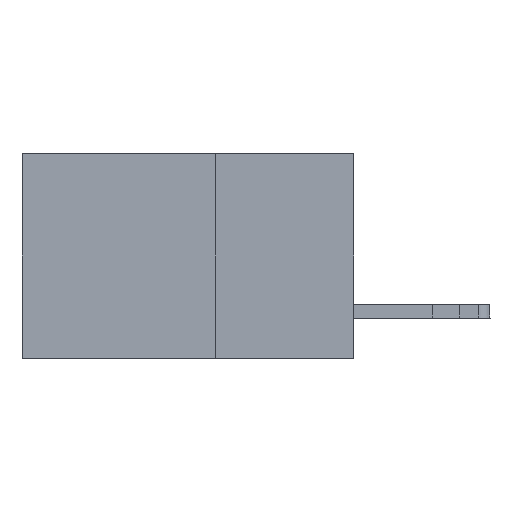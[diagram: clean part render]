
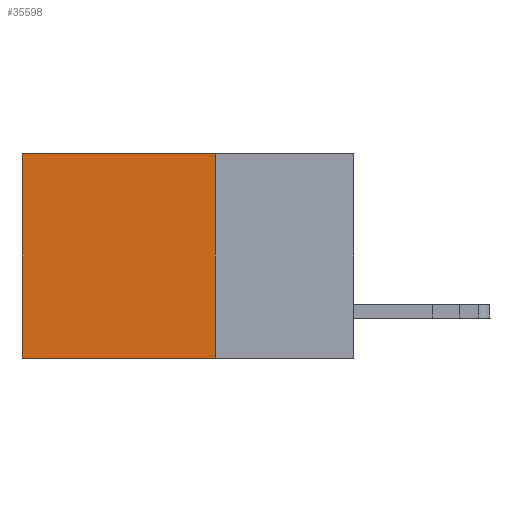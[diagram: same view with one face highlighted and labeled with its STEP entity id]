
A CAD part, left-side view. The second image highlights one B-rep face of the part: STEP entity #35598.
In plain terms, the highlighted planar face has unit normal (-1, 0, 0).
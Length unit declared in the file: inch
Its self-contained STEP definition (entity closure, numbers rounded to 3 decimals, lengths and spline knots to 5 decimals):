
#1536 = ORIENTED_EDGE ( 'NONE', *, *, #14249, .T. ) ;
#2337 = FACE_OUTER_BOUND ( 'NONE', #29533, .T. ) ;
#3650 = EDGE_CURVE ( 'NONE', #5836, #28011, #3689, .T. ) ;
#3689 = LINE ( 'NONE', #14919, #21063 ) ;
#4201 = CARTESIAN_POINT ( 'NONE',  ( 0.2875, 0.6, 0. ) ) ;
#5027 = DIRECTION ( 'NONE',  ( 0., 1., 0. ) ) ;
#5836 = VERTEX_POINT ( 'NONE', #15743 ) ;
#6299 = CARTESIAN_POINT ( 'NONE',  ( 0.2875, 0.6, -0.37 ) ) ;
#6421 = LINE ( 'NONE', #4201, #14195 ) ;
#7461 = LINE ( 'NONE', #18708, #13590 ) ;
#8395 = CARTESIAN_POINT ( 'NONE',  ( 0.2875, 0.6, 0. ) ) ;
#10395 = DIRECTION ( 'NONE',  ( 0., 1., 0. ) ) ;
#11360 = PLANE ( 'NONE',  #32153 ) ;
#12779 = VERTEX_POINT ( 'NONE', #6299 ) ;
#13589 = DIRECTION ( 'NONE',  ( 1., 0., 0. ) ) ;
#13590 = VECTOR ( 'NONE', #10395, 39.37008 ) ;
#14195 = VECTOR ( 'NONE', #18210, 39.37008 ) ;
#14249 = EDGE_CURVE ( 'NONE', #5836, #17093, #27367, .T. ) ;
#14919 = CARTESIAN_POINT ( 'NONE',  ( 0.2875, 0.25, 0. ) ) ;
#15743 = CARTESIAN_POINT ( 'NONE',  ( 0.2875, 0.25, 0. ) ) ;
#16173 = EDGE_CURVE ( 'NONE', #28011, #12779, #7461, .T. ) ;
#16502 = ORIENTED_EDGE ( 'NONE', *, *, #30148, .T. ) ;
#17093 = VERTEX_POINT ( 'NONE', #8395 ) ;
#18210 = DIRECTION ( 'NONE',  ( 0., 0., -1. ) ) ;
#18708 = CARTESIAN_POINT ( 'NONE',  ( 0.2875, 0.25, -0.37 ) ) ;
#20835 = DIRECTION ( 'NONE',  ( 0., 0., -1. ) ) ;
#21063 = VECTOR ( 'NONE', #20835, 39.37008 ) ;
#22638 = CARTESIAN_POINT ( 'NONE',  ( 0.2875, 0.25, 0. ) ) ;
#24214 = CARTESIAN_POINT ( 'NONE',  ( 0.2875, 0.25, 0. ) ) ;
#27367 = LINE ( 'NONE', #24214, #30703 ) ;
#28011 = VERTEX_POINT ( 'NONE', #34847 ) ;
#29533 = EDGE_LOOP ( 'NONE', ( #16502, #32319, #35992, #1536 ) ) ;
#30148 = EDGE_CURVE ( 'NONE', #17093, #12779, #6421, .T. ) ;
#30703 = VECTOR ( 'NONE', #5027, 39.37008 ) ;
#32153 = AXIS2_PLACEMENT_3D ( 'NONE', #22638, #13589, #33719 ) ;
#32319 = ORIENTED_EDGE ( 'NONE', *, *, #16173, .F. ) ;
#33719 = DIRECTION ( 'NONE',  ( 0., 0., -1. ) ) ;
#34847 = CARTESIAN_POINT ( 'NONE',  ( 0.2875, 0.25, -0.37 ) ) ;
#35598 = ADVANCED_FACE ( 'NONE', ( #2337 ), #11360, .F. ) ;
#35992 = ORIENTED_EDGE ( 'NONE', *, *, #3650, .F. ) ;
